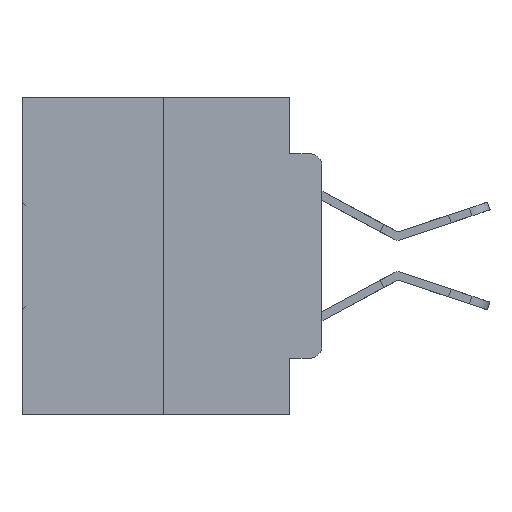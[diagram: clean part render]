
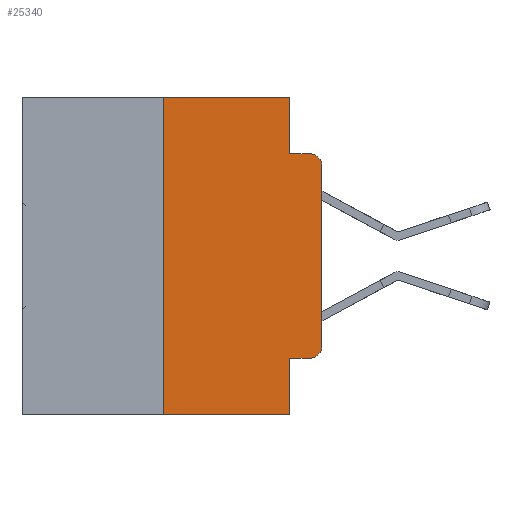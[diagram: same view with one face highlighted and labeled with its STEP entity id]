
A CAD part, left-side view. The second image highlights one B-rep face of the part: STEP entity #25340.
In plain terms, the highlighted planar face has unit normal (-1, 0, 0).
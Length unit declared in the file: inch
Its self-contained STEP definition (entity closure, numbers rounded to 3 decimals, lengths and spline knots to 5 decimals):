
#1297 = EDGE_CURVE ( 'NONE', #6653, #9986, #31451, .T. ) ;
#1474 = CARTESIAN_POINT ( 'NONE',  ( 0., 0.051, 0. ) ) ;
#2569 = CARTESIAN_POINT ( 'NONE',  ( 0., 0.051, 0. ) ) ;
#3950 = CARTESIAN_POINT ( 'NONE',  ( 0., 0.051, -0.0885 ) ) ;
#4790 = CARTESIAN_POINT ( 'NONE',  ( 0., 0.051, -0.4115 ) ) ;
#4909 = VECTOR ( 'NONE', #19565, 39.37008 ) ;
#5402 = CARTESIAN_POINT ( 'NONE',  ( 0., 0.051, 0. ) ) ;
#5619 = ORIENTED_EDGE ( 'NONE', *, *, #20940, .T. ) ;
#5977 = EDGE_CURVE ( 'NONE', #9427, #15497, #27314, .T. ) ;
#6046 = LINE ( 'NONE', #5402, #18622 ) ;
#6653 = VERTEX_POINT ( 'NONE', #3950 ) ;
#7690 = AXIS2_PLACEMENT_3D ( 'NONE', #23044, #8008, #25528 ) ;
#7744 = VECTOR ( 'NONE', #19998, 39.37008 ) ;
#7960 = DIRECTION ( 'NONE',  ( 0., 0., -1. ) ) ;
#8008 = DIRECTION ( 'NONE',  ( -1., 0., 0. ) ) ;
#8796 = VECTOR ( 'NONE', #10298, 39.37008 ) ;
#9029 = CARTESIAN_POINT ( 'NONE',  ( 0., 0.02, -0.4115 ) ) ;
#9322 = LINE ( 'NONE', #9959, #7744 ) ;
#9427 = VERTEX_POINT ( 'NONE', #9871 ) ;
#9871 = CARTESIAN_POINT ( 'NONE',  ( 0., 0.25, -0.5 ) ) ;
#9959 = CARTESIAN_POINT ( 'NONE',  ( 0., 0.473, 0. ) ) ;
#9986 = VERTEX_POINT ( 'NONE', #31963 ) ;
#10298 = DIRECTION ( 'NONE',  ( 0., 0., 1. ) ) ;
#10384 = ORIENTED_EDGE ( 'NONE', *, *, #14338, .T. ) ;
#10647 = EDGE_CURVE ( 'NONE', #31652, #15497, #17911, .T. ) ;
#10806 = ORIENTED_EDGE ( 'NONE', *, *, #5977, .T. ) ;
#11159 = CARTESIAN_POINT ( 'NONE',  ( 0., 0.473, -0.5 ) ) ;
#11942 = ORIENTED_EDGE ( 'NONE', *, *, #1297, .F. ) ;
#12056 = CARTESIAN_POINT ( 'NONE',  ( 0., 0.02, -0.3915 ) ) ;
#12653 = VERTEX_POINT ( 'NONE', #16135 ) ;
#13501 = DIRECTION ( 'NONE',  ( 1., 0., 0. ) ) ;
#14262 = LINE ( 'NONE', #21033, #26719 ) ;
#14306 = ORIENTED_EDGE ( 'NONE', *, *, #21041, .F. ) ;
#14338 = EDGE_CURVE ( 'NONE', #25296, #9986, #21965, .T. ) ;
#14595 = DIRECTION ( 'NONE',  ( 0., 0., -1. ) ) ;
#14867 = VECTOR ( 'NONE', #28571, 39.37008 ) ;
#15362 = EDGE_LOOP ( 'NONE', ( #29452, #10384, #11942, #18578, #14306, #20928, #10806, #24070, #31337, #5619 ) ) ;
#15497 = VERTEX_POINT ( 'NONE', #28684 ) ;
#15514 = LINE ( 'NONE', #17720, #8796 ) ;
#15677 = VECTOR ( 'NONE', #16559, 39.37008 ) ;
#16135 = CARTESIAN_POINT ( 'NONE',  ( 0., 0.25, 0. ) ) ;
#16169 = VERTEX_POINT ( 'NONE', #31802 ) ;
#16443 = LINE ( 'NONE', #26475, #15677 ) ;
#16559 = DIRECTION ( 'NONE',  ( 0., -1., 0. ) ) ;
#16997 = EDGE_CURVE ( 'NONE', #16169, #25296, #15514, .T. ) ;
#17720 = CARTESIAN_POINT ( 'NONE',  ( 0., 0., 0. ) ) ;
#17911 = LINE ( 'NONE', #2569, #23784 ) ;
#18164 = CARTESIAN_POINT ( 'NONE',  ( 0., 0., -0.1085 ) ) ;
#18344 = CIRCLE ( 'NONE', #28015, 0.02 ) ;
#18578 = ORIENTED_EDGE ( 'NONE', *, *, #27060, .F. ) ;
#18622 = VECTOR ( 'NONE', #7960, 39.37008 ) ;
#19565 = DIRECTION ( 'NONE',  ( 0., -1., 0. ) ) ;
#19998 = DIRECTION ( 'NONE',  ( 0., -1., 0. ) ) ;
#20259 = EDGE_CURVE ( 'NONE', #31652, #27325, #16443, .T. ) ;
#20928 = ORIENTED_EDGE ( 'NONE', *, *, #28313, .F. ) ;
#20940 = EDGE_CURVE ( 'NONE', #27325, #16169, #18344, .T. ) ;
#21033 = CARTESIAN_POINT ( 'NONE',  ( 0., 0.25, 0. ) ) ;
#21041 = EDGE_CURVE ( 'NONE', #12653, #25557, #9322, .T. ) ;
#21965 = CIRCLE ( 'NONE', #7690, 0.02 ) ;
#22094 = CARTESIAN_POINT ( 'NONE',  ( 0., 0.051, -0.0885 ) ) ;
#22101 = AXIS2_PLACEMENT_3D ( 'NONE', #28374, #13501, #30827 ) ;
#22816 = DIRECTION ( 'NONE',  ( 0., 0., -1. ) ) ;
#23044 = CARTESIAN_POINT ( 'NONE',  ( 0., 0.02, -0.1085 ) ) ;
#23065 = FACE_OUTER_BOUND ( 'NONE', #15362, .T. ) ;
#23784 = VECTOR ( 'NONE', #22816, 39.37008 ) ;
#24070 = ORIENTED_EDGE ( 'NONE', *, *, #10647, .F. ) ;
#25296 = VERTEX_POINT ( 'NONE', #18164 ) ;
#25340 = ADVANCED_FACE ( 'NONE', ( #23065 ), #25902, .F. ) ;
#25528 = DIRECTION ( 'NONE',  ( 0., 0., -1. ) ) ;
#25557 = VERTEX_POINT ( 'NONE', #1474 ) ;
#25902 = PLANE ( 'NONE',  #22101 ) ;
#26475 = CARTESIAN_POINT ( 'NONE',  ( 0., 0.051, -0.4115 ) ) ;
#26719 = VECTOR ( 'NONE', #30869, 39.37008 ) ;
#27060 = EDGE_CURVE ( 'NONE', #25557, #6653, #6046, .T. ) ;
#27314 = LINE ( 'NONE', #11159, #14867 ) ;
#27325 = VERTEX_POINT ( 'NONE', #9029 ) ;
#28015 = AXIS2_PLACEMENT_3D ( 'NONE', #12056, #29451, #14595 ) ;
#28313 = EDGE_CURVE ( 'NONE', #9427, #12653, #14262, .T. ) ;
#28374 = CARTESIAN_POINT ( 'NONE',  ( 0., 0.473, 0. ) ) ;
#28571 = DIRECTION ( 'NONE',  ( 0., -1., 0. ) ) ;
#28684 = CARTESIAN_POINT ( 'NONE',  ( 0., 0.051, -0.5 ) ) ;
#29451 = DIRECTION ( 'NONE',  ( -1., 0., 0. ) ) ;
#29452 = ORIENTED_EDGE ( 'NONE', *, *, #16997, .T. ) ;
#30827 = DIRECTION ( 'NONE',  ( 0., 0., -1. ) ) ;
#30869 = DIRECTION ( 'NONE',  ( 0., 0., 1. ) ) ;
#31337 = ORIENTED_EDGE ( 'NONE', *, *, #20259, .T. ) ;
#31451 = LINE ( 'NONE', #22094, #4909 ) ;
#31652 = VERTEX_POINT ( 'NONE', #4790 ) ;
#31802 = CARTESIAN_POINT ( 'NONE',  ( 0., 0., -0.3915 ) ) ;
#31963 = CARTESIAN_POINT ( 'NONE',  ( 0., 0.02, -0.0885 ) ) ;
